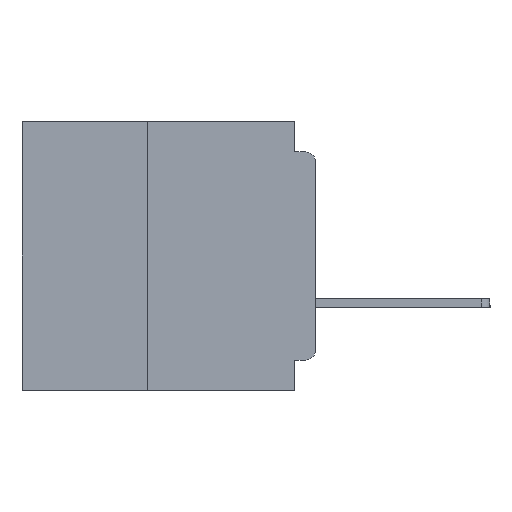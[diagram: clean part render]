
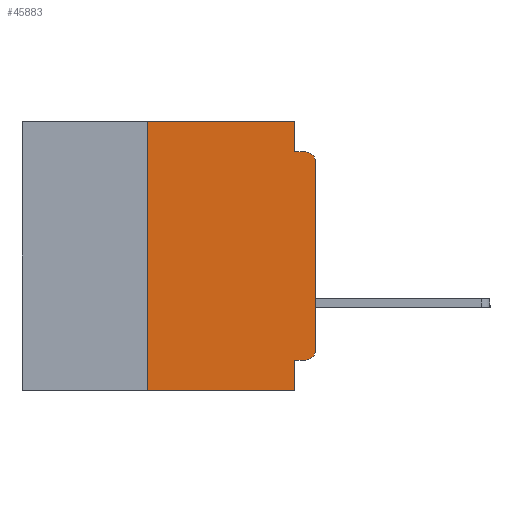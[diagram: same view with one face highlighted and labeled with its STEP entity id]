
A CAD part, left-side view. The second image highlights one B-rep face of the part: STEP entity #45883.
In plain terms, the highlighted planar face has unit normal (-1, 0, 0).
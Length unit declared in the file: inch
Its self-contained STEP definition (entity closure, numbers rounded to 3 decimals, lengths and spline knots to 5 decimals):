
#327 = DIRECTION ( 'NONE',  ( 0., 0., -1. ) ) ;
#1131 = ORIENTED_EDGE ( 'NONE', *, *, #35250, .F. ) ;
#1470 = DIRECTION ( 'NONE',  ( 0., 0., -1. ) ) ;
#2275 = DIRECTION ( 'NONE',  ( 0., 0., -1. ) ) ;
#2506 = DIRECTION ( 'NONE',  ( 0., 0., 1. ) ) ;
#2602 = VERTEX_POINT ( 'NONE', #27942 ) ;
#3091 = CARTESIAN_POINT ( 'NONE',  ( 0., 0.015, -0.045 ) ) ;
#3320 = DIRECTION ( 'NONE',  ( 0., 0., 1. ) ) ;
#3335 = CIRCLE ( 'NONE', #8533, 0.015 ) ;
#3405 = CARTESIAN_POINT ( 'NONE',  ( 0., 0.437, 0. ) ) ;
#8292 = EDGE_CURVE ( 'NONE', #16608, #28268, #38384, .T. ) ;
#8386 = EDGE_CURVE ( 'NONE', #16608, #39121, #10265, .T. ) ;
#8533 = AXIS2_PLACEMENT_3D ( 'NONE', #51309, #25082, #55694 ) ;
#10265 = LINE ( 'NONE', #14047, #57025 ) ;
#10389 = CARTESIAN_POINT ( 'NONE',  ( 0., 0.25, -0.4 ) ) ;
#10637 = LINE ( 'NONE', #21039, #30013 ) ;
#10712 = LINE ( 'NONE', #11316, #56064 ) ;
#11316 = CARTESIAN_POINT ( 'NONE',  ( 0., 0., 0. ) ) ;
#11689 = LINE ( 'NONE', #3405, #22096 ) ;
#11716 = ORIENTED_EDGE ( 'NONE', *, *, #53911, .F. ) ;
#11895 = CARTESIAN_POINT ( 'NONE',  ( 0., 0.031, -0.045 ) ) ;
#12919 = VECTOR ( 'NONE', #2275, 39.37008 ) ;
#14047 = CARTESIAN_POINT ( 'NONE',  ( 0., 0., -0.355 ) ) ;
#14126 = VECTOR ( 'NONE', #22198, 39.37008 ) ;
#14289 = CARTESIAN_POINT ( 'NONE',  ( 0., 0.031, -0.4 ) ) ;
#16239 = EDGE_CURVE ( 'NONE', #26917, #21091, #53035, .T. ) ;
#16608 = VERTEX_POINT ( 'NONE', #36244 ) ;
#17720 = CARTESIAN_POINT ( 'NONE',  ( 0., 0.031, 0. ) ) ;
#17978 = VERTEX_POINT ( 'NONE', #45694 ) ;
#18965 = VERTEX_POINT ( 'NONE', #14289 ) ;
#20480 = EDGE_CURVE ( 'NONE', #35503, #18965, #26930, .T. ) ;
#20500 = CARTESIAN_POINT ( 'NONE',  ( 0., 0.437, -0.4 ) ) ;
#20712 = ORIENTED_EDGE ( 'NONE', *, *, #40633, .T. ) ;
#21039 = CARTESIAN_POINT ( 'NONE',  ( 0., 0.25, -0.4 ) ) ;
#21091 = VERTEX_POINT ( 'NONE', #3091 ) ;
#21188 = ORIENTED_EDGE ( 'NONE', *, *, #20480, .T. ) ;
#22096 = VECTOR ( 'NONE', #56179, 39.37008 ) ;
#22198 = DIRECTION ( 'NONE',  ( 0., 0., -1. ) ) ;
#22929 = CARTESIAN_POINT ( 'NONE',  ( 0., 0.031, -0.355 ) ) ;
#23695 = CARTESIAN_POINT ( 'NONE',  ( 0., 0.437, 0. ) ) ;
#23855 = EDGE_LOOP ( 'NONE', ( #20712, #50488, #49803, #35877, #53042, #1131, #21188, #11716, #28373, #44645 ) ) ;
#24755 = DIRECTION ( 'NONE',  ( 0., -1., 0. ) ) ;
#25082 = DIRECTION ( 'NONE',  ( -1., 0., 0. ) ) ;
#26153 = EDGE_CURVE ( 'NONE', #17978, #21091, #3335, .T. ) ;
#26917 = VERTEX_POINT ( 'NONE', #11895 ) ;
#26930 = LINE ( 'NONE', #20500, #48862 ) ;
#27013 = DIRECTION ( 'NONE',  ( -1., 0., 0. ) ) ;
#27942 = CARTESIAN_POINT ( 'NONE',  ( 0., 0.031, 0. ) ) ;
#28138 = DIRECTION ( 'NONE',  ( 1., 0., 0. ) ) ;
#28268 = VERTEX_POINT ( 'NONE', #43157 ) ;
#28373 = ORIENTED_EDGE ( 'NONE', *, *, #8386, .F. ) ;
#30013 = VECTOR ( 'NONE', #3320, 39.37008 ) ;
#31910 = EDGE_CURVE ( 'NONE', #50266, #2602, #11689, .T. ) ;
#35250 = EDGE_CURVE ( 'NONE', #35503, #50266, #10637, .T. ) ;
#35503 = VERTEX_POINT ( 'NONE', #10389 ) ;
#35795 = CARTESIAN_POINT ( 'NONE',  ( 0., 0.25, 0. ) ) ;
#35877 = ORIENTED_EDGE ( 'NONE', *, *, #41141, .F. ) ;
#36226 = DIRECTION ( 'NONE',  ( 0., 1., 0. ) ) ;
#36244 = CARTESIAN_POINT ( 'NONE',  ( 0., 0.015, -0.355 ) ) ;
#38384 = CIRCLE ( 'NONE', #41436, 0.015 ) ;
#38934 = LINE ( 'NONE', #17720, #14126 ) ;
#39121 = VERTEX_POINT ( 'NONE', #22929 ) ;
#40633 = EDGE_CURVE ( 'NONE', #28268, #17978, #10712, .T. ) ;
#41141 = EDGE_CURVE ( 'NONE', #2602, #26917, #38934, .T. ) ;
#41436 = AXIS2_PLACEMENT_3D ( 'NONE', #53219, #27013, #327 ) ;
#41456 = VECTOR ( 'NONE', #24755, 39.37008 ) ;
#41916 = AXIS2_PLACEMENT_3D ( 'NONE', #23695, #28138, #1470 ) ;
#43157 = CARTESIAN_POINT ( 'NONE',  ( 0., 0., -0.34 ) ) ;
#44645 = ORIENTED_EDGE ( 'NONE', *, *, #8292, .T. ) ;
#45609 = PLANE ( 'NONE',  #41916 ) ;
#45694 = CARTESIAN_POINT ( 'NONE',  ( 0., 0., -0.06 ) ) ;
#45883 = ADVANCED_FACE ( 'NONE', ( #51967 ), #45609, .F. ) ;
#46630 = CARTESIAN_POINT ( 'NONE',  ( 0., 0., -0.045 ) ) ;
#46840 = DIRECTION ( 'NONE',  ( 0., -1., 0. ) ) ;
#48044 = LINE ( 'NONE', #55085, #12919 ) ;
#48862 = VECTOR ( 'NONE', #46840, 39.37008 ) ;
#49803 = ORIENTED_EDGE ( 'NONE', *, *, #16239, .F. ) ;
#50266 = VERTEX_POINT ( 'NONE', #35795 ) ;
#50488 = ORIENTED_EDGE ( 'NONE', *, *, #26153, .T. ) ;
#51309 = CARTESIAN_POINT ( 'NONE',  ( 0., 0.015, -0.06 ) ) ;
#51967 = FACE_OUTER_BOUND ( 'NONE', #23855, .T. ) ;
#53035 = LINE ( 'NONE', #46630, #41456 ) ;
#53042 = ORIENTED_EDGE ( 'NONE', *, *, #31910, .F. ) ;
#53219 = CARTESIAN_POINT ( 'NONE',  ( 0., 0.015, -0.34 ) ) ;
#53911 = EDGE_CURVE ( 'NONE', #39121, #18965, #48044, .T. ) ;
#55085 = CARTESIAN_POINT ( 'NONE',  ( 0., 0.031, -0.4 ) ) ;
#55694 = DIRECTION ( 'NONE',  ( 0., 0., -1. ) ) ;
#56064 = VECTOR ( 'NONE', #2506, 39.37008 ) ;
#56179 = DIRECTION ( 'NONE',  ( 0., -1., 0. ) ) ;
#57025 = VECTOR ( 'NONE', #36226, 39.37008 ) ;
